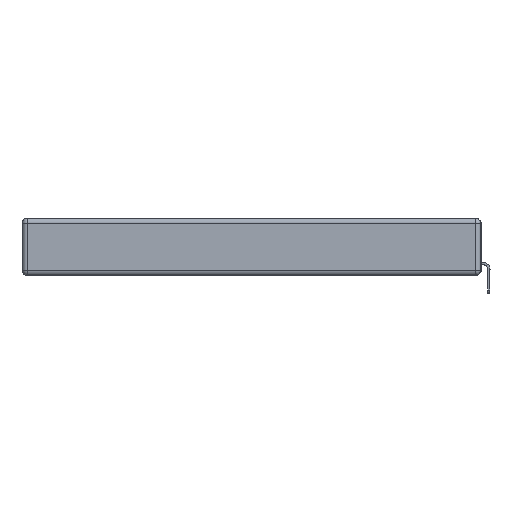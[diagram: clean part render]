
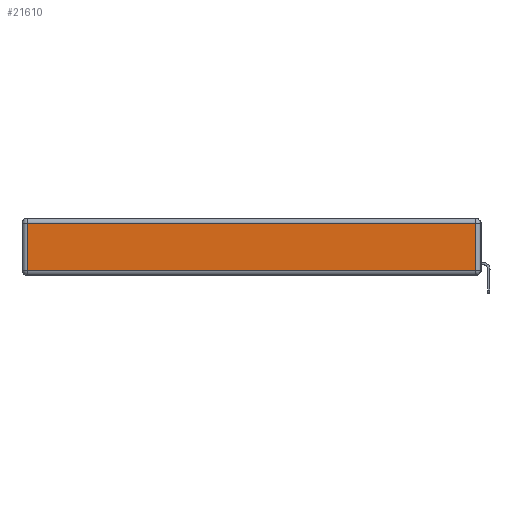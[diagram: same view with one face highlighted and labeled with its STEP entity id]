
A CAD part, left-side view. The second image highlights one B-rep face of the part: STEP entity #21610.
In plain terms, the highlighted planar face has unit normal (-1, 0, 0).
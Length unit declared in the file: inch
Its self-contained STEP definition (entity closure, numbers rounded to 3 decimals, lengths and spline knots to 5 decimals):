
#437 = LINE ( 'NONE', #25150, #19941 ) ;
#937 = CARTESIAN_POINT ( 'NONE',  ( 0., 2.72, -0.343 ) ) ;
#1318 = ORIENTED_EDGE ( 'NONE', *, *, #22072, .T. ) ;
#1421 = LINE ( 'NONE', #20116, #8363 ) ;
#1510 = VERTEX_POINT ( 'NONE', #22979 ) ;
#5322 = EDGE_LOOP ( 'NONE', ( #1318, #19629, #16785, #15073 ) ) ;
#5622 = EDGE_CURVE ( 'NONE', #17663, #21991, #1421, .T. ) ;
#6731 = DIRECTION ( 'NONE',  ( 0., 0., 1. ) ) ;
#8083 = DIRECTION ( 'NONE',  ( 0., 0., 1. ) ) ;
#8363 = VECTOR ( 'NONE', #8083, 39.37008 ) ;
#9019 = EDGE_CURVE ( 'NONE', #21991, #19659, #10210, .T. ) ;
#9616 = VECTOR ( 'NONE', #20230, 39.37008 ) ;
#9953 = CARTESIAN_POINT ( 'NONE',  ( 0., 2.72, -0.03 ) ) ;
#10180 = EDGE_CURVE ( 'NONE', #19659, #1510, #21484, .T. ) ;
#10210 = LINE ( 'NONE', #22520, #9616 ) ;
#10449 = CARTESIAN_POINT ( 'NONE',  ( 0., 0., -0.343 ) ) ;
#14545 = VECTOR ( 'NONE', #21364, 39.37008 ) ;
#14828 = DIRECTION ( 'NONE',  ( 0., -1., 0. ) ) ;
#15073 = ORIENTED_EDGE ( 'NONE', *, *, #10180, .T. ) ;
#16785 = ORIENTED_EDGE ( 'NONE', *, *, #9019, .T. ) ;
#16855 = FACE_OUTER_BOUND ( 'NONE', #5322, .T. ) ;
#17078 = CARTESIAN_POINT ( 'NONE',  ( 0., 0.03, -0.313 ) ) ;
#17391 = AXIS2_PLACEMENT_3D ( 'NONE', #10449, #23154, #6731 ) ;
#17663 = VERTEX_POINT ( 'NONE', #17078 ) ;
#19629 = ORIENTED_EDGE ( 'NONE', *, *, #5622, .T. ) ;
#19659 = VERTEX_POINT ( 'NONE', #9953 ) ;
#19941 = VECTOR ( 'NONE', #14828, 39.37008 ) ;
#20116 = CARTESIAN_POINT ( 'NONE',  ( 0., 0.03, -0.343 ) ) ;
#20230 = DIRECTION ( 'NONE',  ( 0., 1., 0. ) ) ;
#21364 = DIRECTION ( 'NONE',  ( 0., 0., -1. ) ) ;
#21484 = LINE ( 'NONE', #937, #14545 ) ;
#21610 = ADVANCED_FACE ( 'NONE', ( #16855 ), #25039, .T. ) ;
#21991 = VERTEX_POINT ( 'NONE', #23957 ) ;
#22072 = EDGE_CURVE ( 'NONE', #1510, #17663, #437, .T. ) ;
#22520 = CARTESIAN_POINT ( 'NONE',  ( 0., 2.75, -0.03 ) ) ;
#22979 = CARTESIAN_POINT ( 'NONE',  ( 0., 2.72, -0.313 ) ) ;
#23154 = DIRECTION ( 'NONE',  ( -1., 0., 0. ) ) ;
#23957 = CARTESIAN_POINT ( 'NONE',  ( 0., 0.03, -0.03 ) ) ;
#25039 = PLANE ( 'NONE',  #17391 ) ;
#25150 = CARTESIAN_POINT ( 'NONE',  ( 0., 0., -0.313 ) ) ;
